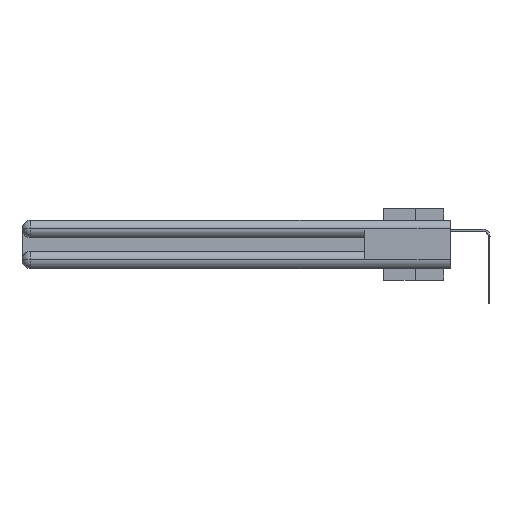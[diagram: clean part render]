
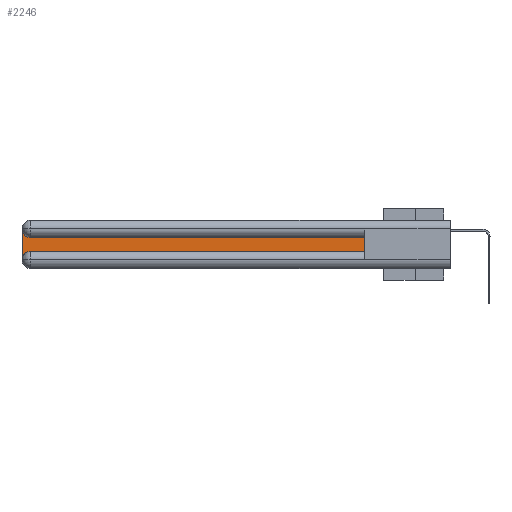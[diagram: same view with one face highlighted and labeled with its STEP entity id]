
A CAD part, left-side view. The second image highlights one B-rep face of the part: STEP entity #2246.
In plain terms, the highlighted planar face has unit normal (-1, 0, 0).
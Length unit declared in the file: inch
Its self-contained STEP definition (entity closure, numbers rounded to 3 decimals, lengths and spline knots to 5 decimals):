
#483 = VERTEX_POINT ( 'NONE', #13410 ) ;
#1258 = AXIS2_PLACEMENT_3D ( 'NONE', #5237, #21281, #19102 ) ;
#1902 = VERTEX_POINT ( 'NONE', #6334 ) ;
#1913 = CARTESIAN_POINT ( 'NONE',  ( 0.075, 0.6, -0.1225 ) ) ;
#2002 = ORIENTED_EDGE ( 'NONE', *, *, #3786, .T. ) ;
#2246 = ADVANCED_FACE ( 'NONE', ( #8678 ), #21177, .F. ) ;
#3110 = CIRCLE ( 'NONE', #26091, 0.06 ) ;
#3786 = EDGE_CURVE ( 'NONE', #13739, #8599, #20169, .T. ) ;
#3908 = AXIS2_PLACEMENT_3D ( 'NONE', #11466, #20417, #25070 ) ;
#4006 = LINE ( 'NONE', #27889, #28029 ) ;
#5237 = CARTESIAN_POINT ( 'NONE',  ( 0.075, 3., -0.1225 ) ) ;
#5496 = CARTESIAN_POINT ( 'NONE',  ( 0.075, 0.6, -0.2175 ) ) ;
#5586 = VECTOR ( 'NONE', #22656, 39.37008 ) ;
#6177 = EDGE_CURVE ( 'NONE', #1902, #28995, #3110, .T. ) ;
#6334 = CARTESIAN_POINT ( 'NONE',  ( 0.075, 3., -0.2775 ) ) ;
#7325 = CARTESIAN_POINT ( 'NONE',  ( 0.075, 2.94, -0.1225 ) ) ;
#8316 = CARTESIAN_POINT ( 'NONE',  ( 0.075, 3., -0.0625 ) ) ;
#8599 = VERTEX_POINT ( 'NONE', #8316 ) ;
#8678 = FACE_OUTER_BOUND ( 'NONE', #24057, .T. ) ;
#9918 = ORIENTED_EDGE ( 'NONE', *, *, #10340, .T. ) ;
#10173 = EDGE_CURVE ( 'NONE', #483, #12575, #4006, .T. ) ;
#10340 = EDGE_CURVE ( 'NONE', #28995, #483, #16691, .T. ) ;
#11466 = CARTESIAN_POINT ( 'NONE',  ( 0.075, 2.94, -0.0625 ) ) ;
#11587 = LINE ( 'NONE', #13481, #5586 ) ;
#11981 = DIRECTION ( 'NONE',  ( 0., 0., -1. ) ) ;
#12032 = ORIENTED_EDGE ( 'NONE', *, *, #6177, .T. ) ;
#12575 = VERTEX_POINT ( 'NONE', #14325 ) ;
#13045 = EDGE_CURVE ( 'NONE', #12575, #13739, #21098, .T. ) ;
#13410 = CARTESIAN_POINT ( 'NONE',  ( 0.075, 0.6, -0.2175 ) ) ;
#13481 = CARTESIAN_POINT ( 'NONE',  ( 0.075, 3., -0.2175 ) ) ;
#13739 = VERTEX_POINT ( 'NONE', #7325 ) ;
#14325 = CARTESIAN_POINT ( 'NONE',  ( 0.075, 0.6, -0.1225 ) ) ;
#14444 = DIRECTION ( 'NONE',  ( 0., 0., 1. ) ) ;
#14520 = CARTESIAN_POINT ( 'NONE',  ( 0.075, 2.94, -0.2175 ) ) ;
#15491 = DIRECTION ( 'NONE',  ( 0., 1., 0. ) ) ;
#16691 = LINE ( 'NONE', #5496, #21287 ) ;
#16777 = DIRECTION ( 'NONE',  ( 1., 0., 0. ) ) ;
#19089 = VECTOR ( 'NONE', #15491, 39.37008 ) ;
#19102 = DIRECTION ( 'NONE',  ( 0., 0., -1. ) ) ;
#20169 = CIRCLE ( 'NONE', #3908, 0.06 ) ;
#20417 = DIRECTION ( 'NONE',  ( 1., 0., 0. ) ) ;
#21098 = LINE ( 'NONE', #1913, #19089 ) ;
#21177 = PLANE ( 'NONE',  #1258 ) ;
#21281 = DIRECTION ( 'NONE',  ( 1., 0., 0. ) ) ;
#21287 = VECTOR ( 'NONE', #28387, 39.37008 ) ;
#22656 = DIRECTION ( 'NONE',  ( 0., 0., -1. ) ) ;
#23123 = ORIENTED_EDGE ( 'NONE', *, *, #13045, .T. ) ;
#24057 = EDGE_LOOP ( 'NONE', ( #23123, #2002, #24459, #12032, #9918, #27069 ) ) ;
#24459 = ORIENTED_EDGE ( 'NONE', *, *, #27101, .T. ) ;
#25070 = DIRECTION ( 'NONE',  ( 0., 0., -1. ) ) ;
#26091 = AXIS2_PLACEMENT_3D ( 'NONE', #27766, #16777, #11981 ) ;
#27069 = ORIENTED_EDGE ( 'NONE', *, *, #10173, .T. ) ;
#27101 = EDGE_CURVE ( 'NONE', #8599, #1902, #11587, .T. ) ;
#27766 = CARTESIAN_POINT ( 'NONE',  ( 0.075, 2.94, -0.2775 ) ) ;
#27889 = CARTESIAN_POINT ( 'NONE',  ( 0.075, 0.6, -0.2175 ) ) ;
#28029 = VECTOR ( 'NONE', #14444, 39.37008 ) ;
#28387 = DIRECTION ( 'NONE',  ( 0., -1., 0. ) ) ;
#28995 = VERTEX_POINT ( 'NONE', #14520 ) ;
